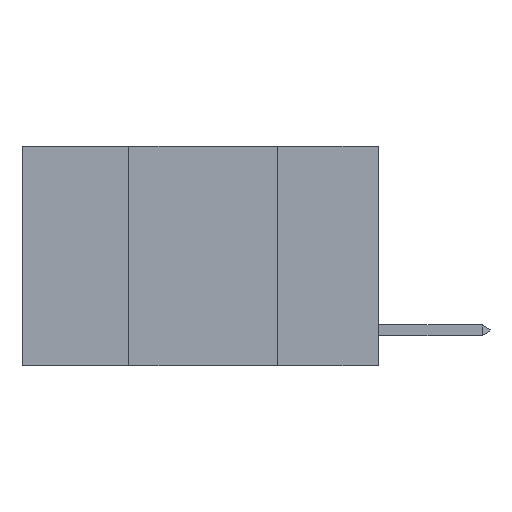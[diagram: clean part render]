
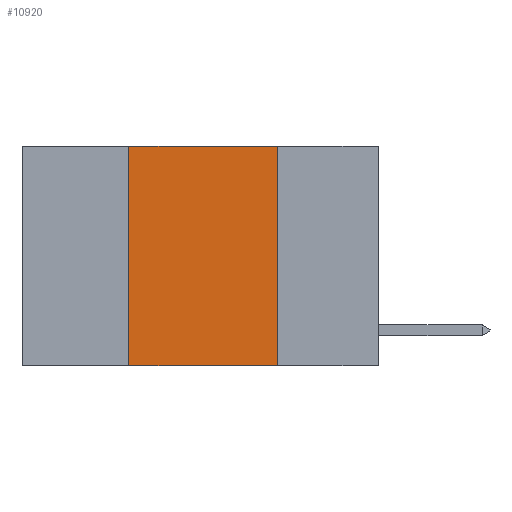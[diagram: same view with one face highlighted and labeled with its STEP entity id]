
A CAD part, left-side view. The second image highlights one B-rep face of the part: STEP entity #10920.
In plain terms, the highlighted planar face has unit normal (-1, 0, 0).
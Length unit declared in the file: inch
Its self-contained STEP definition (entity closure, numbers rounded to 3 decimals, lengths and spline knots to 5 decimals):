
#251 = AXIS2_PLACEMENT_3D ( 'NONE', #12949, #7715, #15814 ) ;
#691 = ORIENTED_EDGE ( 'NONE', *, *, #2472, .F. ) ;
#718 = FACE_OUTER_BOUND ( 'NONE', #16571, .T. ) ;
#862 = CARTESIAN_POINT ( 'NONE',  ( 0., 0.42, -0.37 ) ) ;
#1573 = LINE ( 'NONE', #16349, #14144 ) ;
#1853 = VERTEX_POINT ( 'NONE', #862 ) ;
#2472 = EDGE_CURVE ( 'NONE', #10250, #6731, #16724, .T. ) ;
#3187 = DIRECTION ( 'NONE',  ( 0., -1., 0. ) ) ;
#3251 = CARTESIAN_POINT ( 'NONE',  ( 0., 0.42, 0. ) ) ;
#3273 = DIRECTION ( 'NONE',  ( 0., 0., 1. ) ) ;
#4641 = CARTESIAN_POINT ( 'NONE',  ( 0., 0.17, 0. ) ) ;
#4824 = ORIENTED_EDGE ( 'NONE', *, *, #4938, .F. ) ;
#4938 = EDGE_CURVE ( 'NONE', #1853, #10250, #11360, .T. ) ;
#6262 = VECTOR ( 'NONE', #3187, 39.37008 ) ;
#6710 = DIRECTION ( 'NONE',  ( 0., -1., 0. ) ) ;
#6731 = VERTEX_POINT ( 'NONE', #15741 ) ;
#7510 = EDGE_CURVE ( 'NONE', #1853, #10770, #1573, .T. ) ;
#7715 = DIRECTION ( 'NONE',  ( 1., 0., 0. ) ) ;
#8427 = VECTOR ( 'NONE', #3273, 39.37008 ) ;
#8576 = LINE ( 'NONE', #4641, #15254 ) ;
#10250 = VERTEX_POINT ( 'NONE', #3251 ) ;
#10435 = ORIENTED_EDGE ( 'NONE', *, *, #10627, .F. ) ;
#10627 = EDGE_CURVE ( 'NONE', #6731, #10770, #8576, .T. ) ;
#10770 = VERTEX_POINT ( 'NONE', #13162 ) ;
#10920 = ADVANCED_FACE ( 'NONE', ( #718 ), #14364, .F. ) ;
#11360 = LINE ( 'NONE', #15461, #8427 ) ;
#12949 = CARTESIAN_POINT ( 'NONE',  ( 0., 0.6, 0. ) ) ;
#12974 = ORIENTED_EDGE ( 'NONE', *, *, #7510, .T. ) ;
#13162 = CARTESIAN_POINT ( 'NONE',  ( 0., 0.17, -0.37 ) ) ;
#14144 = VECTOR ( 'NONE', #6710, 39.37008 ) ;
#14364 = PLANE ( 'NONE',  #251 ) ;
#15102 = CARTESIAN_POINT ( 'NONE',  ( 0., 0.6, 0. ) ) ;
#15254 = VECTOR ( 'NONE', #17124, 39.37008 ) ;
#15461 = CARTESIAN_POINT ( 'NONE',  ( 0., 0.42, 0. ) ) ;
#15741 = CARTESIAN_POINT ( 'NONE',  ( 0., 0.17, 0. ) ) ;
#15814 = DIRECTION ( 'NONE',  ( 0., 0., -1. ) ) ;
#16349 = CARTESIAN_POINT ( 'NONE',  ( 0., 0.6, -0.37 ) ) ;
#16571 = EDGE_LOOP ( 'NONE', ( #10435, #691, #4824, #12974 ) ) ;
#16724 = LINE ( 'NONE', #15102, #6262 ) ;
#17124 = DIRECTION ( 'NONE',  ( 0., 0., -1. ) ) ;
